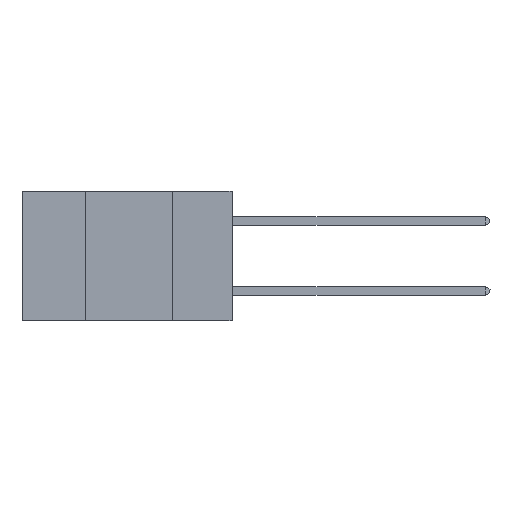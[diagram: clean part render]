
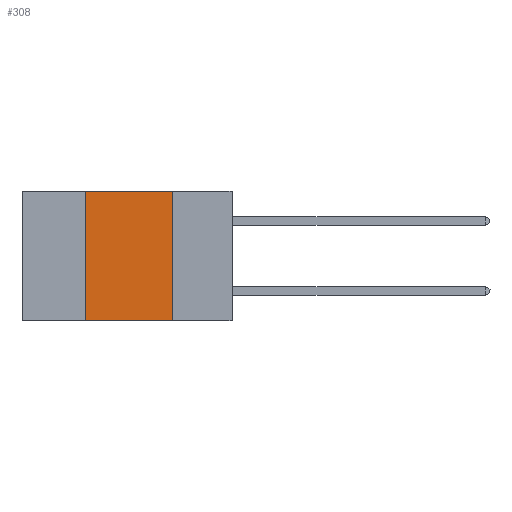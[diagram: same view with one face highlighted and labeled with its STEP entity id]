
A CAD part, left-side view. The second image highlights one B-rep face of the part: STEP entity #308.
In plain terms, the highlighted planar face has unit normal (-1, 0, 0).
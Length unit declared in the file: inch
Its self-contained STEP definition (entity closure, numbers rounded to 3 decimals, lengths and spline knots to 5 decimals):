
#251 = VECTOR ( 'NONE', #9235, 39.37008 ) ;
#308 = ADVANCED_FACE ( 'NONE', ( #2909 ), #772, .F. ) ;
#772 = PLANE ( 'NONE',  #4498 ) ;
#1120 = EDGE_CURVE ( 'NONE', #5538, #9682, #12628, .T. ) ;
#1227 = CARTESIAN_POINT ( 'NONE',  ( 0., 0.6, 0. ) ) ;
#1382 = LINE ( 'NONE', #7521, #11857 ) ;
#1552 = DIRECTION ( 'NONE',  ( 0., 0., 1. ) ) ;
#2015 = CARTESIAN_POINT ( 'NONE',  ( 0., 0.17, -0.37 ) ) ;
#2404 = CARTESIAN_POINT ( 'NONE',  ( 0., 0.42, 0. ) ) ;
#2675 = EDGE_CURVE ( 'NONE', #3653, #12659, #8226, .T. ) ;
#2829 = EDGE_LOOP ( 'NONE', ( #3728, #8572, #10784, #8855 ) ) ;
#2837 = CARTESIAN_POINT ( 'NONE',  ( 0., 0.6, 0. ) ) ;
#2909 = FACE_OUTER_BOUND ( 'NONE', #2829, .T. ) ;
#3653 = VERTEX_POINT ( 'NONE', #2404 ) ;
#3728 = ORIENTED_EDGE ( 'NONE', *, *, #8219, .F. ) ;
#3994 = VECTOR ( 'NONE', #10841, 39.37008 ) ;
#4498 = AXIS2_PLACEMENT_3D ( 'NONE', #2837, #5770, #9842 ) ;
#5538 = VERTEX_POINT ( 'NONE', #11496 ) ;
#5770 = DIRECTION ( 'NONE',  ( 1., 0., 0. ) ) ;
#5783 = CARTESIAN_POINT ( 'NONE',  ( 0., 0.6, -0.37 ) ) ;
#5802 = CARTESIAN_POINT ( 'NONE',  ( 0., 0.17, 0. ) ) ;
#6679 = VECTOR ( 'NONE', #11736, 39.37008 ) ;
#7521 = CARTESIAN_POINT ( 'NONE',  ( 0., 0.42, 0. ) ) ;
#8092 = EDGE_CURVE ( 'NONE', #5538, #3653, #1382, .T. ) ;
#8219 = EDGE_CURVE ( 'NONE', #12659, #9682, #12334, .T. ) ;
#8226 = LINE ( 'NONE', #1227, #251 ) ;
#8572 = ORIENTED_EDGE ( 'NONE', *, *, #2675, .F. ) ;
#8855 = ORIENTED_EDGE ( 'NONE', *, *, #1120, .T. ) ;
#9235 = DIRECTION ( 'NONE',  ( 0., -1., 0. ) ) ;
#9642 = CARTESIAN_POINT ( 'NONE',  ( 0., 0.17, 0. ) ) ;
#9682 = VERTEX_POINT ( 'NONE', #2015 ) ;
#9842 = DIRECTION ( 'NONE',  ( 0., 0., -1. ) ) ;
#10784 = ORIENTED_EDGE ( 'NONE', *, *, #8092, .F. ) ;
#10841 = DIRECTION ( 'NONE',  ( 0., -1., 0. ) ) ;
#11496 = CARTESIAN_POINT ( 'NONE',  ( 0., 0.42, -0.37 ) ) ;
#11736 = DIRECTION ( 'NONE',  ( 0., 0., -1. ) ) ;
#11857 = VECTOR ( 'NONE', #1552, 39.37008 ) ;
#12334 = LINE ( 'NONE', #5802, #6679 ) ;
#12628 = LINE ( 'NONE', #5783, #3994 ) ;
#12659 = VERTEX_POINT ( 'NONE', #9642 ) ;
